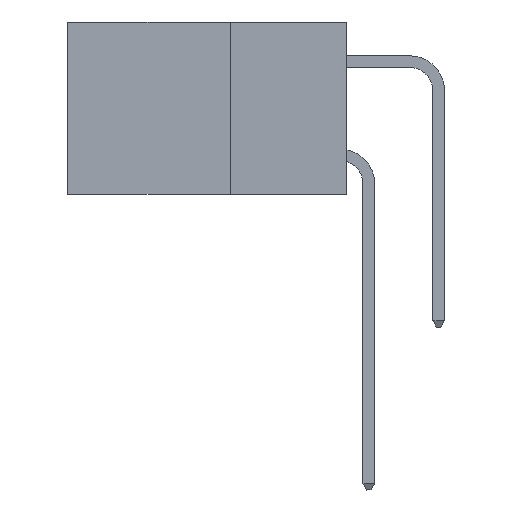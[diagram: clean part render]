
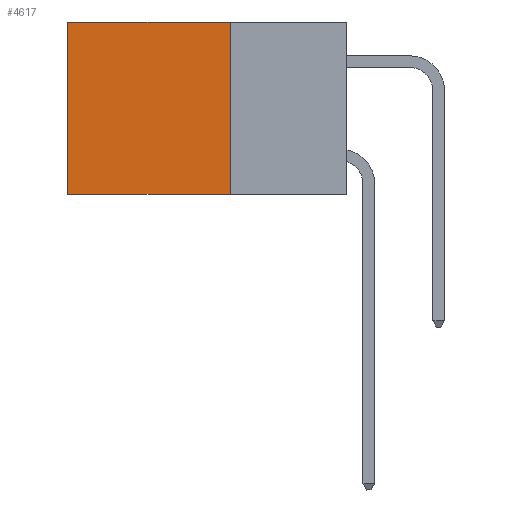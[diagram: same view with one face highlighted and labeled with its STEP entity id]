
A CAD part, left-side view. The second image highlights one B-rep face of the part: STEP entity #4617.
In plain terms, the highlighted planar face has unit normal (-1, 0, 0).
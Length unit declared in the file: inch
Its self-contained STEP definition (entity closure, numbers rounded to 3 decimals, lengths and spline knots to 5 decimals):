
#770 = CARTESIAN_POINT ( 'NONE',  ( 0.2875, 0.6, 0. ) ) ;
#896 = EDGE_LOOP ( 'NONE', ( #27605, #9677, #26612, #20905 ) ) ;
#2474 = LINE ( 'NONE', #26203, #31199 ) ;
#2598 = VECTOR ( 'NONE', #19765, 39.37008 ) ;
#3014 = VERTEX_POINT ( 'NONE', #22607 ) ;
#3373 = DIRECTION ( 'NONE',  ( 1., 0., 0. ) ) ;
#4469 = VERTEX_POINT ( 'NONE', #12553 ) ;
#4617 = ADVANCED_FACE ( 'NONE', ( #23127 ), #14022, .F. ) ;
#5393 = VERTEX_POINT ( 'NONE', #770 ) ;
#7263 = VERTEX_POINT ( 'NONE', #10790 ) ;
#9250 = CARTESIAN_POINT ( 'NONE',  ( 0.2875, 0.6, 0. ) ) ;
#9677 = ORIENTED_EDGE ( 'NONE', *, *, #19566, .F. ) ;
#10706 = DIRECTION ( 'NONE',  ( 0., 1., 0. ) ) ;
#10790 = CARTESIAN_POINT ( 'NONE',  ( 0.2875, 0.25, 0. ) ) ;
#11533 = LINE ( 'NONE', #29161, #12345 ) ;
#12315 = EDGE_CURVE ( 'NONE', #7263, #5393, #24904, .T. ) ;
#12345 = VECTOR ( 'NONE', #10706, 39.37008 ) ;
#12553 = CARTESIAN_POINT ( 'NONE',  ( 0.2875, 0.25, -0.37 ) ) ;
#13024 = EDGE_CURVE ( 'NONE', #7263, #4469, #2474, .T. ) ;
#13250 = LINE ( 'NONE', #9250, #2598 ) ;
#13466 = AXIS2_PLACEMENT_3D ( 'NONE', #27016, #3373, #19299 ) ;
#14022 = PLANE ( 'NONE',  #13466 ) ;
#17291 = EDGE_CURVE ( 'NONE', #5393, #3014, #13250, .T. ) ;
#18485 = DIRECTION ( 'NONE',  ( 0., 0., -1. ) ) ;
#19299 = DIRECTION ( 'NONE',  ( 0., 0., -1. ) ) ;
#19566 = EDGE_CURVE ( 'NONE', #4469, #3014, #11533, .T. ) ;
#19765 = DIRECTION ( 'NONE',  ( 0., 0., -1. ) ) ;
#20905 = ORIENTED_EDGE ( 'NONE', *, *, #12315, .T. ) ;
#22607 = CARTESIAN_POINT ( 'NONE',  ( 0.2875, 0.6, -0.37 ) ) ;
#23127 = FACE_OUTER_BOUND ( 'NONE', #896, .T. ) ;
#24904 = LINE ( 'NONE', #25014, #30572 ) ;
#25014 = CARTESIAN_POINT ( 'NONE',  ( 0.2875, 0.25, 0. ) ) ;
#26203 = CARTESIAN_POINT ( 'NONE',  ( 0.2875, 0.25, 0. ) ) ;
#26612 = ORIENTED_EDGE ( 'NONE', *, *, #13024, .F. ) ;
#27016 = CARTESIAN_POINT ( 'NONE',  ( 0.2875, 0.25, 0. ) ) ;
#27605 = ORIENTED_EDGE ( 'NONE', *, *, #17291, .T. ) ;
#29161 = CARTESIAN_POINT ( 'NONE',  ( 0.2875, 0.25, -0.37 ) ) ;
#30460 = DIRECTION ( 'NONE',  ( 0., 1., 0. ) ) ;
#30572 = VECTOR ( 'NONE', #30460, 39.37008 ) ;
#31199 = VECTOR ( 'NONE', #18485, 39.37008 ) ;
